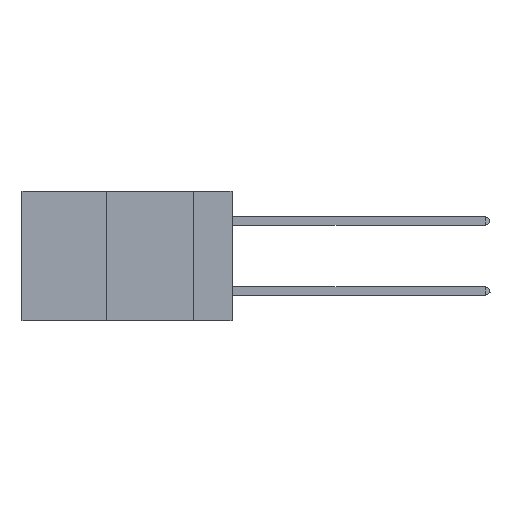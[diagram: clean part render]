
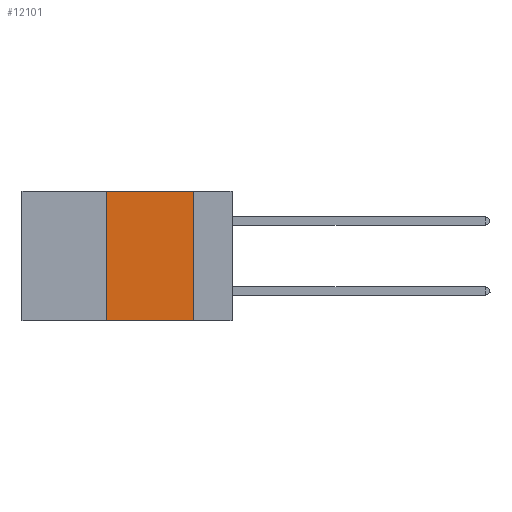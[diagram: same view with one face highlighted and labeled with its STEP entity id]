
A CAD part, left-side view. The second image highlights one B-rep face of the part: STEP entity #12101.
In plain terms, the highlighted planar face has unit normal (-1, 0, 0).
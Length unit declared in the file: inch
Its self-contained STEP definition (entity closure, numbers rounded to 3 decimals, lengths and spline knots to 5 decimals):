
#643 = VERTEX_POINT ( 'NONE', #13602 ) ;
#857 = VECTOR ( 'NONE', #4288, 39.37008 ) ;
#1300 = EDGE_CURVE ( 'NONE', #14770, #10594, #8652, .T. ) ;
#1827 = LINE ( 'NONE', #16808, #857 ) ;
#1934 = CARTESIAN_POINT ( 'NONE',  ( 0., 0.6, 0. ) ) ;
#2053 = DIRECTION ( 'NONE',  ( 0., 0., -1. ) ) ;
#2273 = CARTESIAN_POINT ( 'NONE',  ( 0., 0.11, 0. ) ) ;
#2580 = FACE_OUTER_BOUND ( 'NONE', #10917, .T. ) ;
#3332 = CARTESIAN_POINT ( 'NONE',  ( 0., 0.36, -0.37 ) ) ;
#3587 = ORIENTED_EDGE ( 'NONE', *, *, #9056, .F. ) ;
#4288 = DIRECTION ( 'NONE',  ( 0., -1., 0. ) ) ;
#6100 = CARTESIAN_POINT ( 'NONE',  ( 0., 0.36, 0. ) ) ;
#6582 = DIRECTION ( 'NONE',  ( 0., -1., 0. ) ) ;
#7016 = CARTESIAN_POINT ( 'NONE',  ( 0., 0.36, 0. ) ) ;
#7139 = AXIS2_PLACEMENT_3D ( 'NONE', #15017, #16543, #15481 ) ;
#7651 = DIRECTION ( 'NONE',  ( 0., 0., 1. ) ) ;
#8652 = LINE ( 'NONE', #1934, #11290 ) ;
#9041 = VECTOR ( 'NONE', #7651, 39.37008 ) ;
#9056 = EDGE_CURVE ( 'NONE', #10594, #643, #15053, .T. ) ;
#10594 = VERTEX_POINT ( 'NONE', #2273 ) ;
#10917 = EDGE_LOOP ( 'NONE', ( #3587, #17841, #18898, #18582 ) ) ;
#11290 = VECTOR ( 'NONE', #6582, 39.37008 ) ;
#11827 = PLANE ( 'NONE',  #7139 ) ;
#12101 = ADVANCED_FACE ( 'NONE', ( #2580 ), #11827, .F. ) ;
#12873 = CARTESIAN_POINT ( 'NONE',  ( 0., 0.11, 0. ) ) ;
#13093 = EDGE_CURVE ( 'NONE', #13839, #14770, #14092, .T. ) ;
#13232 = EDGE_CURVE ( 'NONE', #13839, #643, #1827, .T. ) ;
#13602 = CARTESIAN_POINT ( 'NONE',  ( 0., 0.11, -0.37 ) ) ;
#13839 = VERTEX_POINT ( 'NONE', #3332 ) ;
#14092 = LINE ( 'NONE', #6100, #9041 ) ;
#14770 = VERTEX_POINT ( 'NONE', #7016 ) ;
#15017 = CARTESIAN_POINT ( 'NONE',  ( 0., 0.6, 0. ) ) ;
#15053 = LINE ( 'NONE', #12873, #17199 ) ;
#15481 = DIRECTION ( 'NONE',  ( 0., 0., -1. ) ) ;
#16543 = DIRECTION ( 'NONE',  ( 1., 0., 0. ) ) ;
#16808 = CARTESIAN_POINT ( 'NONE',  ( 0., 0.6, -0.37 ) ) ;
#17199 = VECTOR ( 'NONE', #2053, 39.37008 ) ;
#17841 = ORIENTED_EDGE ( 'NONE', *, *, #1300, .F. ) ;
#18582 = ORIENTED_EDGE ( 'NONE', *, *, #13232, .T. ) ;
#18898 = ORIENTED_EDGE ( 'NONE', *, *, #13093, .F. ) ;
